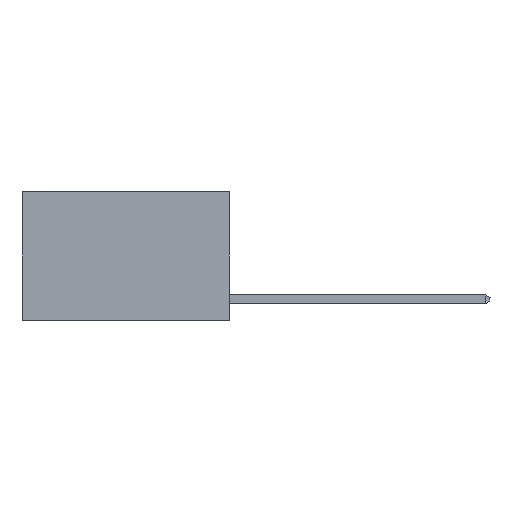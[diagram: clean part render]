
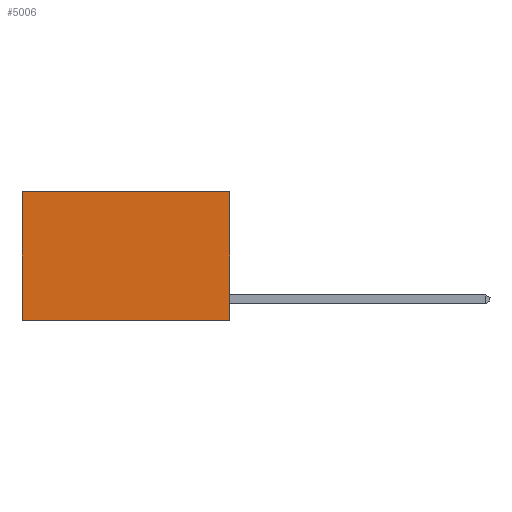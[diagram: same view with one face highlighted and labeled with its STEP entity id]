
A CAD part, left-side view. The second image highlights one B-rep face of the part: STEP entity #5006.
In plain terms, the highlighted planar face has unit normal (-1, 0, 0).
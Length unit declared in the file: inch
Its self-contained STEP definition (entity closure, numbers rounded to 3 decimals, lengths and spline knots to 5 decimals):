
#41 = CARTESIAN_POINT ( 'NONE',  ( 0.2625, 0.6, -0.37 ) ) ;
#760 = DIRECTION ( 'NONE',  ( 1., 0., 0. ) ) ;
#846 = VECTOR ( 'NONE', #17352, 39.37008 ) ;
#1141 = EDGE_CURVE ( 'NONE', #27372, #18211, #8731, .T. ) ;
#1613 = CARTESIAN_POINT ( 'NONE',  ( 0.2625, 0., 0. ) ) ;
#4677 = CARTESIAN_POINT ( 'NONE',  ( 0.2625, 0., -0.37 ) ) ;
#4768 = ORIENTED_EDGE ( 'NONE', *, *, #1141, .T. ) ;
#4922 = FACE_OUTER_BOUND ( 'NONE', #7866, .T. ) ;
#5006 = ADVANCED_FACE ( 'NONE', ( #4922 ), #13933, .F. ) ;
#5949 = DIRECTION ( 'NONE',  ( 0., 0., -1. ) ) ;
#6067 = DIRECTION ( 'NONE',  ( 0., 1., 0. ) ) ;
#7866 = EDGE_LOOP ( 'NONE', ( #12546, #10620, #17207, #4768 ) ) ;
#8337 = LINE ( 'NONE', #10697, #846 ) ;
#8731 = LINE ( 'NONE', #1613, #15123 ) ;
#8952 = VERTEX_POINT ( 'NONE', #4677 ) ;
#10620 = ORIENTED_EDGE ( 'NONE', *, *, #21606, .F. ) ;
#10697 = CARTESIAN_POINT ( 'NONE',  ( 0.2625, 0.6, 0. ) ) ;
#11720 = VECTOR ( 'NONE', #17102, 39.37008 ) ;
#12546 = ORIENTED_EDGE ( 'NONE', *, *, #22296, .T. ) ;
#13196 = CARTESIAN_POINT ( 'NONE',  ( 0.2625, 0., 0. ) ) ;
#13933 = PLANE ( 'NONE',  #23563 ) ;
#14958 = CARTESIAN_POINT ( 'NONE',  ( 0.2625, 0., 0. ) ) ;
#15123 = VECTOR ( 'NONE', #6067, 39.37008 ) ;
#17102 = DIRECTION ( 'NONE',  ( 0., 0., -1. ) ) ;
#17207 = ORIENTED_EDGE ( 'NONE', *, *, #23163, .F. ) ;
#17352 = DIRECTION ( 'NONE',  ( 0., 0., -1. ) ) ;
#18211 = VERTEX_POINT ( 'NONE', #29006 ) ;
#18298 = CARTESIAN_POINT ( 'NONE',  ( 0.2625, 0., -0.37 ) ) ;
#19456 = CARTESIAN_POINT ( 'NONE',  ( 0.2625, 0., 0. ) ) ;
#20503 = LINE ( 'NONE', #18298, #21583 ) ;
#21583 = VECTOR ( 'NONE', #27300, 39.37008 ) ;
#21606 = EDGE_CURVE ( 'NONE', #8952, #26411, #20503, .T. ) ;
#22296 = EDGE_CURVE ( 'NONE', #18211, #26411, #8337, .T. ) ;
#23163 = EDGE_CURVE ( 'NONE', #27372, #8952, #28177, .T. ) ;
#23563 = AXIS2_PLACEMENT_3D ( 'NONE', #14958, #760, #5949 ) ;
#26411 = VERTEX_POINT ( 'NONE', #41 ) ;
#27300 = DIRECTION ( 'NONE',  ( 0., 1., 0. ) ) ;
#27372 = VERTEX_POINT ( 'NONE', #13196 ) ;
#28177 = LINE ( 'NONE', #19456, #11720 ) ;
#29006 = CARTESIAN_POINT ( 'NONE',  ( 0.2625, 0.6, 0. ) ) ;
